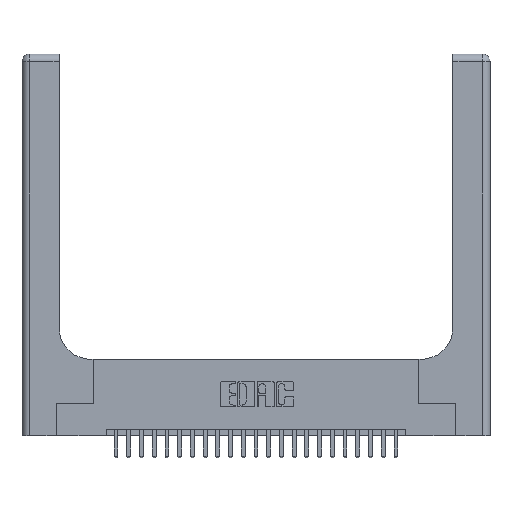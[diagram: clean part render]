
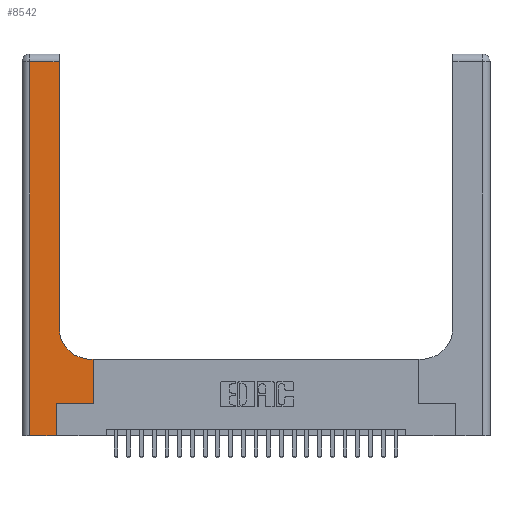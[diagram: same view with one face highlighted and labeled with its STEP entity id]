
A CAD part, top view. The second image highlights one B-rep face of the part: STEP entity #8542.
In plain terms, the highlighted planar face has unit normal (0, 0, 1).
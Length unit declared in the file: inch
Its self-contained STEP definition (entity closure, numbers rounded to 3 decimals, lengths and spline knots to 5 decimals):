
#16 = CARTESIAN_POINT ( 'NONE',  ( 0.5585, 0.25, 0.37 ) ) ;
#382 = CARTESIAN_POINT ( 'NONE',  ( 0.06, 2.94, 0.37 ) ) ;
#499 = EDGE_CURVE ( 'NONE', #1706, #16809, #10123, .T. ) ;
#690 = DIRECTION ( 'NONE',  ( 0., 1., 0. ) ) ;
#1115 = ORIENTED_EDGE ( 'NONE', *, *, #25457, .T. ) ;
#1388 = ORIENTED_EDGE ( 'NONE', *, *, #24671, .T. ) ;
#1486 = LINE ( 'NONE', #19053, #22904 ) ;
#1543 = CARTESIAN_POINT ( 'NONE',  ( 0.269, 0., 0.37 ) ) ;
#1544 = ORIENTED_EDGE ( 'NONE', *, *, #4166, .T. ) ;
#1706 = VERTEX_POINT ( 'NONE', #9213 ) ;
#3940 = ORIENTED_EDGE ( 'NONE', *, *, #22503, .T. ) ;
#4166 = EDGE_CURVE ( 'NONE', #8755, #1706, #18477, .T. ) ;
#4377 = LINE ( 'NONE', #12333, #15281 ) ;
#4681 = VECTOR ( 'NONE', #14197, 39.37008 ) ;
#5309 = FACE_OUTER_BOUND ( 'NONE', #15406, .T. ) ;
#6046 = ORIENTED_EDGE ( 'NONE', *, *, #8227, .T. ) ;
#7006 = CARTESIAN_POINT ( 'NONE',  ( 0., 3., 0.37 ) ) ;
#7828 = CARTESIAN_POINT ( 'NONE',  ( 0., 0., 0.37 ) ) ;
#7852 = DIRECTION ( 'NONE',  ( 0., 0., -1. ) ) ;
#8207 = LINE ( 'NONE', #17323, #18983 ) ;
#8227 = EDGE_CURVE ( 'NONE', #9160, #17727, #4377, .T. ) ;
#8542 = ADVANCED_FACE ( 'NONE', ( #5309 ), #17189, .F. ) ;
#8645 = VERTEX_POINT ( 'NONE', #19375 ) ;
#8755 = VERTEX_POINT ( 'NONE', #23464 ) ;
#9121 = DIRECTION ( 'NONE',  ( -1., 0., 0. ) ) ;
#9160 = VERTEX_POINT ( 'NONE', #382 ) ;
#9213 = CARTESIAN_POINT ( 'NONE',  ( 0.2915, 0.85, 0.37 ) ) ;
#10123 = LINE ( 'NONE', #14463, #10787 ) ;
#10787 = VECTOR ( 'NONE', #14531, 39.37008 ) ;
#11190 = DIRECTION ( 'NONE',  ( -1., 0., 0. ) ) ;
#11705 = CARTESIAN_POINT ( 'NONE',  ( 0.5585, 0.6, 0.37 ) ) ;
#12010 = VERTEX_POINT ( 'NONE', #16 ) ;
#12333 = CARTESIAN_POINT ( 'NONE',  ( 0.06, 3., 0.37 ) ) ;
#12466 = EDGE_CURVE ( 'NONE', #8645, #12010, #19342, .T. ) ;
#12713 = VECTOR ( 'NONE', #21841, 39.37008 ) ;
#13097 = CARTESIAN_POINT ( 'NONE',  ( 0.5585, 0.25, 0.37 ) ) ;
#13256 = EDGE_CURVE ( 'NONE', #14702, #8645, #1486, .T. ) ;
#13511 = VECTOR ( 'NONE', #15867, 39.37008 ) ;
#13530 = AXIS2_PLACEMENT_3D ( 'NONE', #7006, #22989, #11190 ) ;
#13709 = ORIENTED_EDGE ( 'NONE', *, *, #16613, .T. ) ;
#13965 = CARTESIAN_POINT ( 'NONE',  ( 0.269, 0.25, 0.37 ) ) ;
#14197 = DIRECTION ( 'NONE',  ( -1., 0., 0. ) ) ;
#14463 = CARTESIAN_POINT ( 'NONE',  ( 0.2915, 3., 0.37 ) ) ;
#14531 = DIRECTION ( 'NONE',  ( 0., 1., 0. ) ) ;
#14702 = VERTEX_POINT ( 'NONE', #1543 ) ;
#15079 = ORIENTED_EDGE ( 'NONE', *, *, #13256, .T. ) ;
#15281 = VECTOR ( 'NONE', #23986, 39.37008 ) ;
#15406 = EDGE_LOOP ( 'NONE', ( #22424, #1115, #6046, #13709, #15079, #21274, #3940, #1388, #1544 ) ) ;
#15696 = LINE ( 'NONE', #13097, #25300 ) ;
#15867 = DIRECTION ( 'NONE',  ( 1., 0., 0. ) ) ;
#16613 = EDGE_CURVE ( 'NONE', #17727, #14702, #22465, .T. ) ;
#16809 = VERTEX_POINT ( 'NONE', #24262 ) ;
#16815 = AXIS2_PLACEMENT_3D ( 'NONE', #19940, #7852, #21870 ) ;
#17189 = PLANE ( 'NONE',  #13530 ) ;
#17323 = CARTESIAN_POINT ( 'NONE',  ( 0.2915, 0.6, 0.37 ) ) ;
#17727 = VERTEX_POINT ( 'NONE', #21544 ) ;
#18136 = CARTESIAN_POINT ( 'NONE',  ( 0., 2.94, 0.37 ) ) ;
#18477 = CIRCLE ( 'NONE', #16815, 0.25 ) ;
#18983 = VECTOR ( 'NONE', #9121, 39.37008 ) ;
#19053 = CARTESIAN_POINT ( 'NONE',  ( 0.269, 0., 0.37 ) ) ;
#19342 = LINE ( 'NONE', #13965, #13511 ) ;
#19375 = CARTESIAN_POINT ( 'NONE',  ( 0.269, 0.25, 0.37 ) ) ;
#19940 = CARTESIAN_POINT ( 'NONE',  ( 0.5415, 0.85, 0.37 ) ) ;
#20161 = LINE ( 'NONE', #18136, #4681 ) ;
#20997 = DIRECTION ( 'NONE',  ( 0., 1., 0. ) ) ;
#21274 = ORIENTED_EDGE ( 'NONE', *, *, #12466, .T. ) ;
#21530 = VERTEX_POINT ( 'NONE', #11705 ) ;
#21544 = CARTESIAN_POINT ( 'NONE',  ( 0.06, 0., 0.37 ) ) ;
#21841 = DIRECTION ( 'NONE',  ( 1., 0., 0. ) ) ;
#21870 = DIRECTION ( 'NONE',  ( 1., 0., 0. ) ) ;
#22424 = ORIENTED_EDGE ( 'NONE', *, *, #499, .T. ) ;
#22465 = LINE ( 'NONE', #7828, #12713 ) ;
#22503 = EDGE_CURVE ( 'NONE', #12010, #21530, #15696, .T. ) ;
#22904 = VECTOR ( 'NONE', #20997, 39.37008 ) ;
#22989 = DIRECTION ( 'NONE',  ( 0., 0., -1. ) ) ;
#23464 = CARTESIAN_POINT ( 'NONE',  ( 0.5415, 0.6, 0.37 ) ) ;
#23986 = DIRECTION ( 'NONE',  ( 0., -1., 0. ) ) ;
#24262 = CARTESIAN_POINT ( 'NONE',  ( 0.2915, 2.94, 0.37 ) ) ;
#24671 = EDGE_CURVE ( 'NONE', #21530, #8755, #8207, .T. ) ;
#25300 = VECTOR ( 'NONE', #690, 39.37008 ) ;
#25457 = EDGE_CURVE ( 'NONE', #16809, #9160, #20161, .T. ) ;
